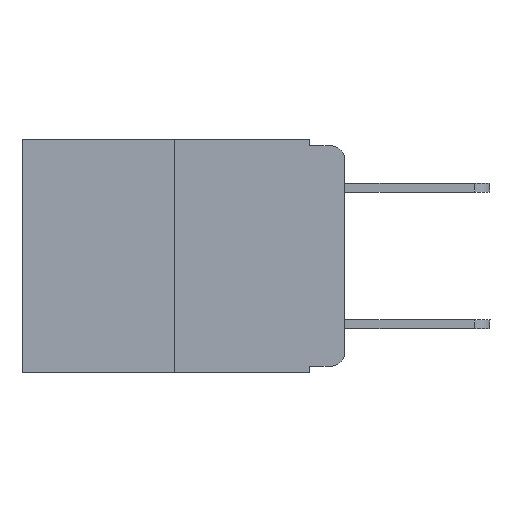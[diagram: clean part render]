
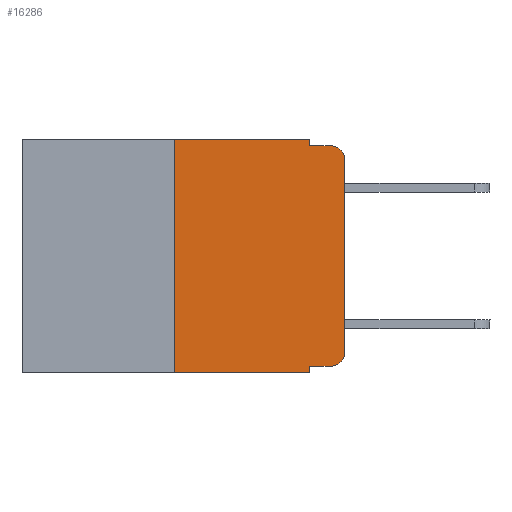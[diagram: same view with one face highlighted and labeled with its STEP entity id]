
A CAD part, left-side view. The second image highlights one B-rep face of the part: STEP entity #16286.
In plain terms, the highlighted planar face has unit normal (-1, 0, 0).
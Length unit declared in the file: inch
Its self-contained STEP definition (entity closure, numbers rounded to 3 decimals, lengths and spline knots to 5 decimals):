
#24 = CARTESIAN_POINT ( 'NONE',  ( 0., 0.25, 0. ) ) ;
#41 = CARTESIAN_POINT ( 'NONE',  ( 0., 0.051, -0.333 ) ) ;
#71 = DIRECTION ( 'NONE',  ( 0., 0., 1. ) ) ;
#106 = VERTEX_POINT ( 'NONE', #6311 ) ;
#311 = EDGE_CURVE ( 'NONE', #15110, #13499, #7099, .T. ) ;
#1023 = CARTESIAN_POINT ( 'NONE',  ( 0., 0.25, 0. ) ) ;
#1141 = CARTESIAN_POINT ( 'NONE',  ( 0., 0.051, 0. ) ) ;
#1751 = EDGE_CURVE ( 'NONE', #13499, #106, #7185, .T. ) ;
#2136 = DIRECTION ( 'NONE',  ( 0., -1., 0. ) ) ;
#2478 = LINE ( 'NONE', #7786, #10753 ) ;
#2693 = ORIENTED_EDGE ( 'NONE', *, *, #6936, .F. ) ;
#2950 = CARTESIAN_POINT ( 'NONE',  ( 0., 0.051, -0.01 ) ) ;
#2975 = DIRECTION ( 'NONE',  ( 0., 0., -1. ) ) ;
#3033 = AXIS2_PLACEMENT_3D ( 'NONE', #12440, #16391, #12594 ) ;
#3555 = VERTEX_POINT ( 'NONE', #15084 ) ;
#3628 = VERTEX_POINT ( 'NONE', #14483 ) ;
#3731 = CARTESIAN_POINT ( 'NONE',  ( 0., 0., -0.03 ) ) ;
#3745 = VERTEX_POINT ( 'NONE', #9596 ) ;
#3750 = DIRECTION ( 'NONE',  ( 0., -1., 0. ) ) ;
#4040 = CARTESIAN_POINT ( 'NONE',  ( 0., 0., 0. ) ) ;
#4066 = CIRCLE ( 'NONE', #12084, 0.02 ) ;
#4509 = DIRECTION ( 'NONE',  ( 0., -1., 0. ) ) ;
#4862 = FACE_OUTER_BOUND ( 'NONE', #8997, .T. ) ;
#5094 = ORIENTED_EDGE ( 'NONE', *, *, #311, .T. ) ;
#5296 = DIRECTION ( 'NONE',  ( 0., 0., 1. ) ) ;
#5501 = ORIENTED_EDGE ( 'NONE', *, *, #1751, .T. ) ;
#6022 = DIRECTION ( 'NONE',  ( 1., 0., 0. ) ) ;
#6075 = LINE ( 'NONE', #10219, #7440 ) ;
#6117 = PLANE ( 'NONE',  #11781 ) ;
#6311 = CARTESIAN_POINT ( 'NONE',  ( 0., 0.02, -0.01 ) ) ;
#6487 = VERTEX_POINT ( 'NONE', #11657 ) ;
#6936 = EDGE_CURVE ( 'NONE', #8508, #6487, #8989, .T. ) ;
#7099 = LINE ( 'NONE', #4040, #11272 ) ;
#7142 = ORIENTED_EDGE ( 'NONE', *, *, #16520, .T. ) ;
#7185 = CIRCLE ( 'NONE', #3033, 0.02 ) ;
#7230 = CARTESIAN_POINT ( 'NONE',  ( 0., 0.473, -0.343 ) ) ;
#7256 = ORIENTED_EDGE ( 'NONE', *, *, #12221, .F. ) ;
#7261 = CARTESIAN_POINT ( 'NONE',  ( 0., 0.473, 0. ) ) ;
#7440 = VECTOR ( 'NONE', #11334, 39.37008 ) ;
#7542 = ORIENTED_EDGE ( 'NONE', *, *, #10063, .F. ) ;
#7582 = EDGE_CURVE ( 'NONE', #3628, #11594, #14440, .T. ) ;
#7605 = CARTESIAN_POINT ( 'NONE',  ( 0., 0.473, 0. ) ) ;
#7786 = CARTESIAN_POINT ( 'NONE',  ( 0., 0.051, 0. ) ) ;
#8307 = VECTOR ( 'NONE', #5296, 39.37008 ) ;
#8508 = VERTEX_POINT ( 'NONE', #1023 ) ;
#8989 = LINE ( 'NONE', #7605, #13657 ) ;
#8997 = EDGE_LOOP ( 'NONE', ( #5094, #5501, #10966, #7542, #2693, #7256, #13100, #15356, #13471, #7142 ) ) ;
#9249 = DIRECTION ( 'NONE',  ( 0., 0., -1. ) ) ;
#9309 = EDGE_CURVE ( 'NONE', #3628, #3555, #10503, .T. ) ;
#9447 = EDGE_CURVE ( 'NONE', #3745, #3555, #12454, .T. ) ;
#9596 = CARTESIAN_POINT ( 'NONE',  ( 0., 0.25, -0.343 ) ) ;
#9750 = DIRECTION ( 'NONE',  ( -1., 0., 0. ) ) ;
#10063 = EDGE_CURVE ( 'NONE', #6487, #13956, #2478, .T. ) ;
#10172 = DIRECTION ( 'NONE',  ( 0., 0., -1. ) ) ;
#10187 = VECTOR ( 'NONE', #4509, 39.37008 ) ;
#10219 = CARTESIAN_POINT ( 'NONE',  ( 0., 0.051, -0.01 ) ) ;
#10503 = LINE ( 'NONE', #1141, #11793 ) ;
#10681 = CARTESIAN_POINT ( 'NONE',  ( 0., 0.02, -0.313 ) ) ;
#10748 = CARTESIAN_POINT ( 'NONE',  ( 0., 0., -0.313 ) ) ;
#10753 = VECTOR ( 'NONE', #9249, 39.37008 ) ;
#10966 = ORIENTED_EDGE ( 'NONE', *, *, #15448, .F. ) ;
#11272 = VECTOR ( 'NONE', #71, 39.37008 ) ;
#11334 = DIRECTION ( 'NONE',  ( 0., -1., 0. ) ) ;
#11594 = VERTEX_POINT ( 'NONE', #15227 ) ;
#11657 = CARTESIAN_POINT ( 'NONE',  ( 0., 0.051, 0. ) ) ;
#11781 = AXIS2_PLACEMENT_3D ( 'NONE', #7261, #6022, #10172 ) ;
#11793 = VECTOR ( 'NONE', #15633, 39.37008 ) ;
#11862 = LINE ( 'NONE', #24, #8307 ) ;
#12084 = AXIS2_PLACEMENT_3D ( 'NONE', #10681, #9750, #2975 ) ;
#12221 = EDGE_CURVE ( 'NONE', #3745, #8508, #11862, .T. ) ;
#12440 = CARTESIAN_POINT ( 'NONE',  ( 0., 0.02, -0.03 ) ) ;
#12454 = LINE ( 'NONE', #7230, #10187 ) ;
#12594 = DIRECTION ( 'NONE',  ( 0., 0., -1. ) ) ;
#13100 = ORIENTED_EDGE ( 'NONE', *, *, #9447, .T. ) ;
#13471 = ORIENTED_EDGE ( 'NONE', *, *, #7582, .T. ) ;
#13499 = VERTEX_POINT ( 'NONE', #3731 ) ;
#13657 = VECTOR ( 'NONE', #2136, 39.37008 ) ;
#13956 = VERTEX_POINT ( 'NONE', #2950 ) ;
#14440 = LINE ( 'NONE', #41, #15888 ) ;
#14483 = CARTESIAN_POINT ( 'NONE',  ( 0., 0.051, -0.333 ) ) ;
#15084 = CARTESIAN_POINT ( 'NONE',  ( 0., 0.051, -0.343 ) ) ;
#15110 = VERTEX_POINT ( 'NONE', #10748 ) ;
#15227 = CARTESIAN_POINT ( 'NONE',  ( 0., 0.02, -0.333 ) ) ;
#15356 = ORIENTED_EDGE ( 'NONE', *, *, #9309, .F. ) ;
#15448 = EDGE_CURVE ( 'NONE', #13956, #106, #6075, .T. ) ;
#15633 = DIRECTION ( 'NONE',  ( 0., 0., -1. ) ) ;
#15888 = VECTOR ( 'NONE', #3750, 39.37008 ) ;
#16286 = ADVANCED_FACE ( 'NONE', ( #4862 ), #6117, .F. ) ;
#16391 = DIRECTION ( 'NONE',  ( -1., 0., 0. ) ) ;
#16520 = EDGE_CURVE ( 'NONE', #11594, #15110, #4066, .T. ) ;
